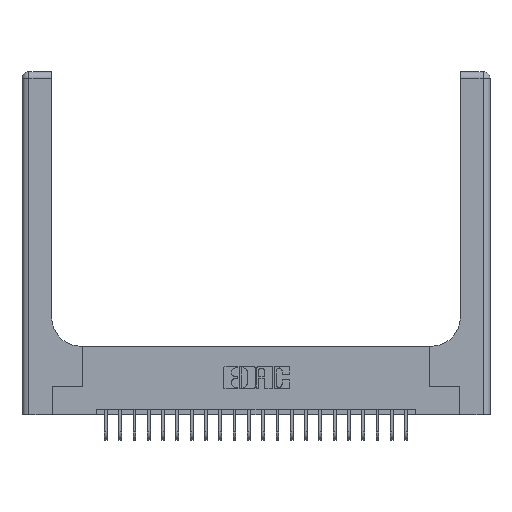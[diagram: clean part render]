
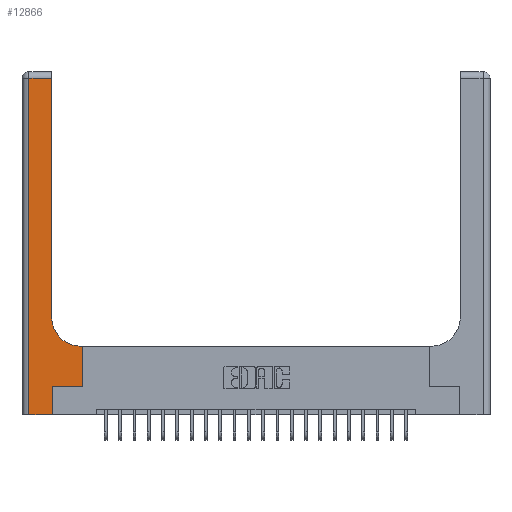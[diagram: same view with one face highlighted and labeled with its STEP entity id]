
A CAD part, top view. The second image highlights one B-rep face of the part: STEP entity #12866.
In plain terms, the highlighted planar face has unit normal (0, 0, 1).
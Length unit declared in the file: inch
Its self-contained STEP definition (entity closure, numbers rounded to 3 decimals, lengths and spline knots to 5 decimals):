
#25 = CARTESIAN_POINT ( 'NONE',  ( 0.528, 0.25, 0.37 ) ) ;
#104 = DIRECTION ( 'NONE',  ( 0., 1., 0. ) ) ;
#108 = CARTESIAN_POINT ( 'NONE',  ( 0.51, 0.6, 0.37 ) ) ;
#256 = VECTOR ( 'NONE', #16583, 39.37008 ) ;
#582 = CARTESIAN_POINT ( 'NONE',  ( 0.265, 0., 0.37 ) ) ;
#1141 = CARTESIAN_POINT ( 'NONE',  ( 0.528, 0.6, 0.37 ) ) ;
#1251 = CARTESIAN_POINT ( 'NONE',  ( 0., 0., 0.37 ) ) ;
#1383 = ORIENTED_EDGE ( 'NONE', *, *, #5015, .T. ) ;
#1541 = VECTOR ( 'NONE', #104, 39.37008 ) ;
#1568 = VERTEX_POINT ( 'NONE', #108 ) ;
#1698 = VECTOR ( 'NONE', #6327, 39.37008 ) ;
#1739 = CARTESIAN_POINT ( 'NONE',  ( 0., 2.94, 0.37 ) ) ;
#1804 = VERTEX_POINT ( 'NONE', #1141 ) ;
#1950 = DIRECTION ( 'NONE',  ( -1., 0., 0. ) ) ;
#2221 = VERTEX_POINT ( 'NONE', #17540 ) ;
#3197 = DIRECTION ( 'NONE',  ( 1., 0., 0. ) ) ;
#3405 = CARTESIAN_POINT ( 'NONE',  ( 0.06, 3., 0.37 ) ) ;
#3876 = PLANE ( 'NONE',  #7055 ) ;
#4251 = VERTEX_POINT ( 'NONE', #19507 ) ;
#4720 = ORIENTED_EDGE ( 'NONE', *, *, #5855, .T. ) ;
#4763 = ORIENTED_EDGE ( 'NONE', *, *, #15958, .T. ) ;
#4878 = VERTEX_POINT ( 'NONE', #23827 ) ;
#5015 = EDGE_CURVE ( 'NONE', #5019, #13948, #10128, .T. ) ;
#5019 = VERTEX_POINT ( 'NONE', #12481 ) ;
#5226 = EDGE_CURVE ( 'NONE', #13934, #4251, #8404, .T. ) ;
#5504 = DIRECTION ( 'NONE',  ( 0., 0., -1. ) ) ;
#5743 = DIRECTION ( 'NONE',  ( -1., 0., 0. ) ) ;
#5855 = EDGE_CURVE ( 'NONE', #1804, #1568, #8957, .T. ) ;
#5932 = EDGE_CURVE ( 'NONE', #1568, #13934, #18858, .T. ) ;
#5979 = CARTESIAN_POINT ( 'NONE',  ( 0.26, 0.6, 0.37 ) ) ;
#6297 = DIRECTION ( 'NONE',  ( 0., 0., -1. ) ) ;
#6327 = DIRECTION ( 'NONE',  ( 1., 0., 0. ) ) ;
#7055 = AXIS2_PLACEMENT_3D ( 'NONE', #14712, #5504, #1950 ) ;
#7868 = LINE ( 'NONE', #3405, #22686 ) ;
#7917 = ORIENTED_EDGE ( 'NONE', *, *, #5932, .T. ) ;
#8404 = LINE ( 'NONE', #17209, #15680 ) ;
#8929 = LINE ( 'NONE', #17455, #1698 ) ;
#8957 = LINE ( 'NONE', #5979, #16530 ) ;
#10126 = ORIENTED_EDGE ( 'NONE', *, *, #22147, .T. ) ;
#10128 = LINE ( 'NONE', #1251, #22941 ) ;
#10589 = EDGE_LOOP ( 'NONE', ( #21117, #4763, #17695, #1383, #13909, #10126, #14542, #4720, #7917 ) ) ;
#10927 = CARTESIAN_POINT ( 'NONE',  ( 0.528, 0.25, 0.37 ) ) ;
#10994 = EDGE_CURVE ( 'NONE', #4878, #5019, #7868, .T. ) ;
#11707 = CARTESIAN_POINT ( 'NONE',  ( 0.51, 0.85, 0.37 ) ) ;
#12481 = CARTESIAN_POINT ( 'NONE',  ( 0.06, 0., 0.37 ) ) ;
#12863 = EDGE_CURVE ( 'NONE', #13948, #2221, #19257, .T. ) ;
#12866 = ADVANCED_FACE ( 'NONE', ( #16052 ), #3876, .F. ) ;
#12988 = DIRECTION ( 'NONE',  ( 0., 1., 0. ) ) ;
#13412 = DIRECTION ( 'NONE',  ( 0., 1., 0. ) ) ;
#13471 = EDGE_CURVE ( 'NONE', #16582, #1804, #16922, .T. ) ;
#13691 = VECTOR ( 'NONE', #12988, 39.37008 ) ;
#13909 = ORIENTED_EDGE ( 'NONE', *, *, #12863, .T. ) ;
#13934 = VERTEX_POINT ( 'NONE', #22654 ) ;
#13948 = VERTEX_POINT ( 'NONE', #582 ) ;
#14459 = DIRECTION ( 'NONE',  ( 0., -1., 0. ) ) ;
#14542 = ORIENTED_EDGE ( 'NONE', *, *, #13471, .T. ) ;
#14712 = CARTESIAN_POINT ( 'NONE',  ( 0., 3., 0.37 ) ) ;
#15680 = VECTOR ( 'NONE', #13412, 39.37008 ) ;
#15958 = EDGE_CURVE ( 'NONE', #4251, #4878, #17692, .T. ) ;
#16052 = FACE_OUTER_BOUND ( 'NONE', #10589, .T. ) ;
#16530 = VECTOR ( 'NONE', #5743, 39.37008 ) ;
#16582 = VERTEX_POINT ( 'NONE', #10927 ) ;
#16583 = DIRECTION ( 'NONE',  ( -1., 0., 0. ) ) ;
#16922 = LINE ( 'NONE', #25, #1541 ) ;
#17209 = CARTESIAN_POINT ( 'NONE',  ( 0.26, 3., 0.37 ) ) ;
#17455 = CARTESIAN_POINT ( 'NONE',  ( 0.265, 0.25, 0.37 ) ) ;
#17540 = CARTESIAN_POINT ( 'NONE',  ( 0.265, 0.25, 0.37 ) ) ;
#17692 = LINE ( 'NONE', #1739, #256 ) ;
#17695 = ORIENTED_EDGE ( 'NONE', *, *, #10994, .T. ) ;
#18858 = CIRCLE ( 'NONE', #22213, 0.25 ) ;
#19257 = LINE ( 'NONE', #22047, #13691 ) ;
#19507 = CARTESIAN_POINT ( 'NONE',  ( 0.26, 2.94, 0.37 ) ) ;
#21117 = ORIENTED_EDGE ( 'NONE', *, *, #5226, .T. ) ;
#22047 = CARTESIAN_POINT ( 'NONE',  ( 0.265, 0., 0.37 ) ) ;
#22147 = EDGE_CURVE ( 'NONE', #2221, #16582, #8929, .T. ) ;
#22213 = AXIS2_PLACEMENT_3D ( 'NONE', #11707, #6297, #22846 ) ;
#22654 = CARTESIAN_POINT ( 'NONE',  ( 0.26, 0.85, 0.37 ) ) ;
#22686 = VECTOR ( 'NONE', #14459, 39.37008 ) ;
#22846 = DIRECTION ( 'NONE',  ( 1., 0., 0. ) ) ;
#22941 = VECTOR ( 'NONE', #3197, 39.37008 ) ;
#23827 = CARTESIAN_POINT ( 'NONE',  ( 0.06, 2.94, 0.37 ) ) ;
